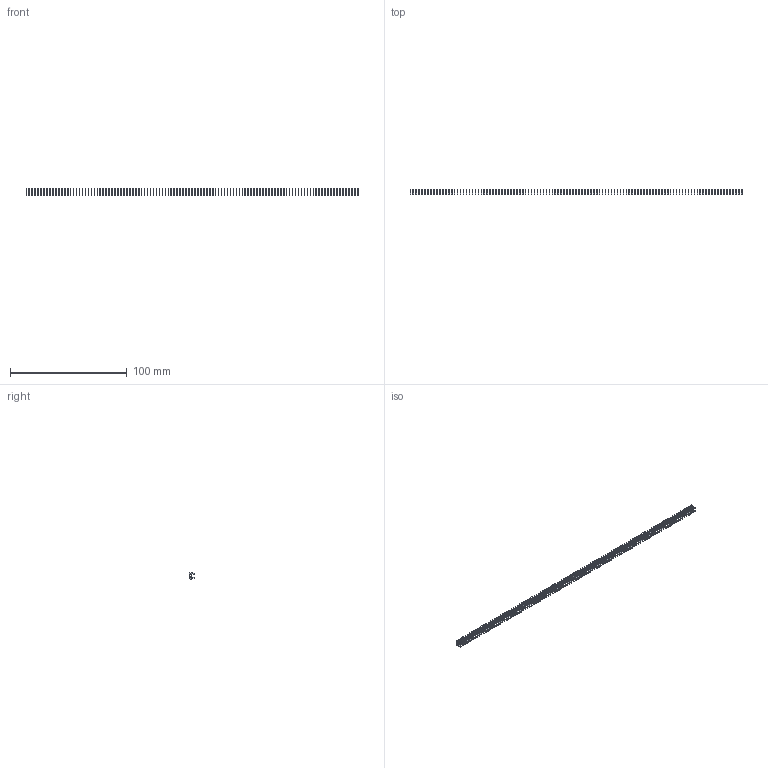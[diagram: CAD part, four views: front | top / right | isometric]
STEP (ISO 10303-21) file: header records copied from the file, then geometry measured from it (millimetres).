
FILE_DESCRIPTION (( 'STEP AP203' ), '1' );
FILE_NAME ('105-113-208-100.STEP', '2020-04-08T01:24:13', ( '' ), ( '' ), 'SwSTEP 2.0', 'SolidWorks 2016', '' );
FILE_SCHEMA (( 'CONFIG_CONTROL_DESIGN' ));
Length unit declared in the file: inch
Products named in the file (2): 105-113-208-100; 100-290-001_100-290-208
Assembly tree (113 placements, depth 2):
  105-113-208-100
    100-290-001_100-290-208  x113
Bounding box: 284.99 x 4.83 x 5.17 mm (x, y, z)
Volume: 777.5 mm3; surface area: 4802.1 mm2
Topology: 113 solids, 113 shells, 2825 faces, 7797 edges, 5198 vertices
Faces by surface type: plane 2486, cylinder 339
Entity records: 4573 total; most frequent: DIRECTION 357, CARTESIAN_POINT 256, DATE_AND_TIME 236, CALENDAR_DATE 236, COORDINATED_UNIVERSAL_TIME_OFFSET 236, LOCAL_TIME 236, AXIS2_PLACEMENT_3D 147, ORIENTED_EDGE 138
